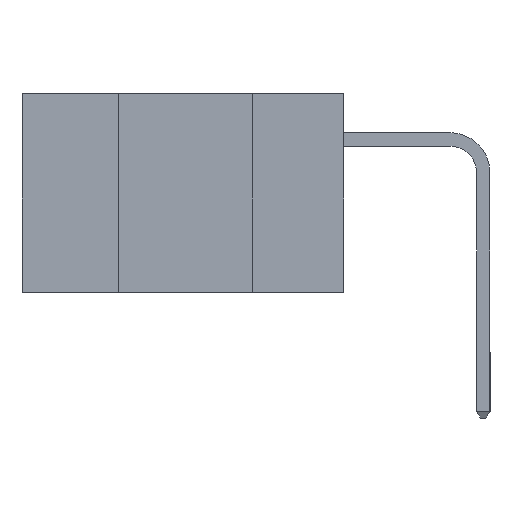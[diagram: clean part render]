
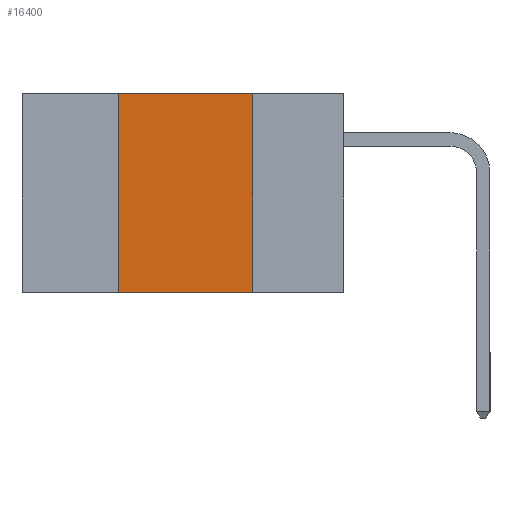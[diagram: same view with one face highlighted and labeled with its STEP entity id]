
A CAD part, left-side view. The second image highlights one B-rep face of the part: STEP entity #16400.
In plain terms, the highlighted planar face has unit normal (-1, 0, 0).
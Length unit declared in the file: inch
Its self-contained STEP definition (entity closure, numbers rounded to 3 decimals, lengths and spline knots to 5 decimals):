
#227 = DIRECTION ( 'NONE',  ( 0., -1., 0. ) ) ;
#864 = ORIENTED_EDGE ( 'NONE', *, *, #15404, .F. ) ;
#972 = PLANE ( 'NONE',  #1609 ) ;
#1609 = AXIS2_PLACEMENT_3D ( 'NONE', #17487, #22119, #23121 ) ;
#2723 = VECTOR ( 'NONE', #227, 39.37008 ) ;
#2799 = ORIENTED_EDGE ( 'NONE', *, *, #19819, .F. ) ;
#5876 = DIRECTION ( 'NONE',  ( 0., -1., 0. ) ) ;
#6138 = DIRECTION ( 'NONE',  ( 0., 0., -1. ) ) ;
#7236 = VECTOR ( 'NONE', #6138, 39.37008 ) ;
#8251 = VECTOR ( 'NONE', #5876, 39.37008 ) ;
#8277 = LINE ( 'NONE', #26256, #24345 ) ;
#8293 = CARTESIAN_POINT ( 'NONE',  ( 0., 0.17, 0. ) ) ;
#8498 = CARTESIAN_POINT ( 'NONE',  ( 0., 0.17, 0. ) ) ;
#10139 = CARTESIAN_POINT ( 'NONE',  ( 0., 0.42, -0.37 ) ) ;
#10224 = DIRECTION ( 'NONE',  ( 0., 0., 1. ) ) ;
#10716 = VERTEX_POINT ( 'NONE', #28482 ) ;
#11087 = EDGE_CURVE ( 'NONE', #14104, #12206, #25447, .T. ) ;
#11817 = ORIENTED_EDGE ( 'NONE', *, *, #16329, .T. ) ;
#12206 = VERTEX_POINT ( 'NONE', #12353 ) ;
#12353 = CARTESIAN_POINT ( 'NONE',  ( 0., 0.17, -0.37 ) ) ;
#14104 = VERTEX_POINT ( 'NONE', #8498 ) ;
#14269 = CARTESIAN_POINT ( 'NONE',  ( 0., 0.6, 0. ) ) ;
#15404 = EDGE_CURVE ( 'NONE', #10716, #14104, #20675, .T. ) ;
#16329 = EDGE_CURVE ( 'NONE', #24361, #12206, #21325, .T. ) ;
#16400 = ADVANCED_FACE ( 'NONE', ( #19146 ), #972, .F. ) ;
#17487 = CARTESIAN_POINT ( 'NONE',  ( 0., 0.6, 0. ) ) ;
#19146 = FACE_OUTER_BOUND ( 'NONE', #26053, .T. ) ;
#19819 = EDGE_CURVE ( 'NONE', #24361, #10716, #8277, .T. ) ;
#20675 = LINE ( 'NONE', #14269, #8251 ) ;
#21325 = LINE ( 'NONE', #25906, #2723 ) ;
#22119 = DIRECTION ( 'NONE',  ( 1., 0., 0. ) ) ;
#23121 = DIRECTION ( 'NONE',  ( 0., 0., -1. ) ) ;
#24345 = VECTOR ( 'NONE', #10224, 39.37008 ) ;
#24361 = VERTEX_POINT ( 'NONE', #10139 ) ;
#25447 = LINE ( 'NONE', #8293, #7236 ) ;
#25906 = CARTESIAN_POINT ( 'NONE',  ( 0., 0.6, -0.37 ) ) ;
#26053 = EDGE_LOOP ( 'NONE', ( #28661, #864, #2799, #11817 ) ) ;
#26256 = CARTESIAN_POINT ( 'NONE',  ( 0., 0.42, 0. ) ) ;
#28482 = CARTESIAN_POINT ( 'NONE',  ( 0., 0.42, 0. ) ) ;
#28661 = ORIENTED_EDGE ( 'NONE', *, *, #11087, .F. ) ;
